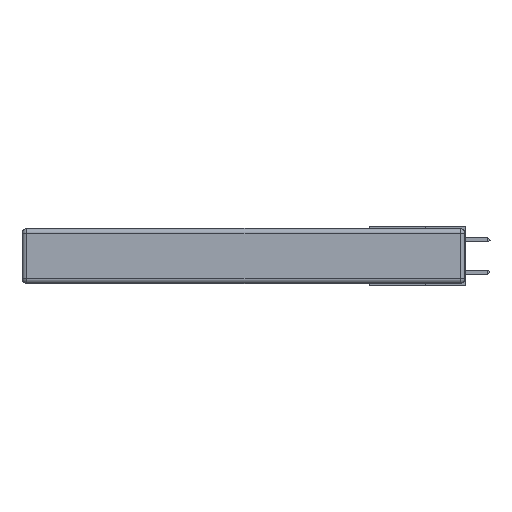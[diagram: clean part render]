
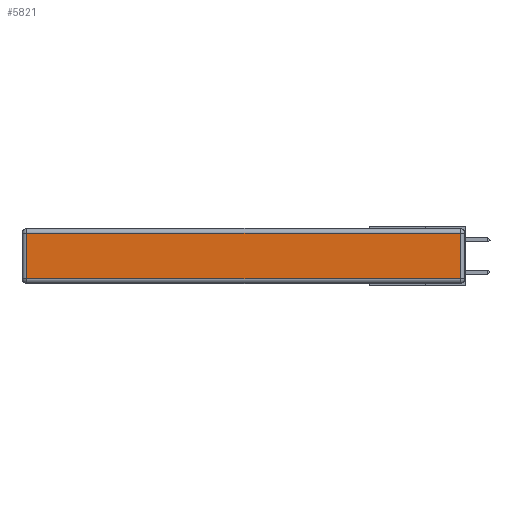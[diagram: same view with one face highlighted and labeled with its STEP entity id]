
A CAD part, left-side view. The second image highlights one B-rep face of the part: STEP entity #5821.
In plain terms, the highlighted planar face has unit normal (-1, 0, 0).
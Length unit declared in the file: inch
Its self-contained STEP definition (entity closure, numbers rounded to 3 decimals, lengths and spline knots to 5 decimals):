
#253 = DIRECTION ( 'NONE',  ( 0., 0., 1. ) ) ;
#642 = ORIENTED_EDGE ( 'NONE', *, *, #15399, .T. ) ;
#1373 = CARTESIAN_POINT ( 'NONE',  ( 0., 0., -0.313 ) ) ;
#1536 = CARTESIAN_POINT ( 'NONE',  ( 0., 0.03, -0.343 ) ) ;
#2411 = LINE ( 'NONE', #11753, #5885 ) ;
#2417 = ORIENTED_EDGE ( 'NONE', *, *, #6206, .T. ) ;
#2902 = DIRECTION ( 'NONE',  ( 0., 0., 1. ) ) ;
#4657 = AXIS2_PLACEMENT_3D ( 'NONE', #5674, #5861, #253 ) ;
#5674 = CARTESIAN_POINT ( 'NONE',  ( 0., 0., -0.343 ) ) ;
#5821 = ADVANCED_FACE ( 'NONE', ( #10409 ), #12538, .T. ) ;
#5861 = DIRECTION ( 'NONE',  ( -1., 0., 0. ) ) ;
#5885 = VECTOR ( 'NONE', #14591, 39.37008 ) ;
#6206 = EDGE_CURVE ( 'NONE', #10304, #14383, #2411, .T. ) ;
#6364 = LINE ( 'NONE', #1536, #15002 ) ;
#7269 = CARTESIAN_POINT ( 'NONE',  ( 0., 2.75, -0.03 ) ) ;
#7339 = ORIENTED_EDGE ( 'NONE', *, *, #17480, .T. ) ;
#7557 = VERTEX_POINT ( 'NONE', #16564 ) ;
#10304 = VERTEX_POINT ( 'NONE', #13798 ) ;
#10409 = FACE_OUTER_BOUND ( 'NONE', #11026, .T. ) ;
#11026 = EDGE_LOOP ( 'NONE', ( #642, #13218, #7339, #2417 ) ) ;
#11340 = EDGE_CURVE ( 'NONE', #7557, #13754, #6364, .T. ) ;
#11575 = CARTESIAN_POINT ( 'NONE',  ( 0., 2.72, -0.313 ) ) ;
#11753 = CARTESIAN_POINT ( 'NONE',  ( 0., 2.72, -0.343 ) ) ;
#12538 = PLANE ( 'NONE',  #4657 ) ;
#13218 = ORIENTED_EDGE ( 'NONE', *, *, #11340, .T. ) ;
#13429 = CARTESIAN_POINT ( 'NONE',  ( 0., 0.03, -0.03 ) ) ;
#13461 = VECTOR ( 'NONE', #14397, 39.37008 ) ;
#13754 = VERTEX_POINT ( 'NONE', #13429 ) ;
#13798 = CARTESIAN_POINT ( 'NONE',  ( 0., 2.72, -0.03 ) ) ;
#14383 = VERTEX_POINT ( 'NONE', #11575 ) ;
#14397 = DIRECTION ( 'NONE',  ( 0., 1., 0. ) ) ;
#14558 = LINE ( 'NONE', #7269, #13461 ) ;
#14591 = DIRECTION ( 'NONE',  ( 0., 0., -1. ) ) ;
#15002 = VECTOR ( 'NONE', #2902, 39.37008 ) ;
#15399 = EDGE_CURVE ( 'NONE', #14383, #7557, #16839, .T. ) ;
#16388 = VECTOR ( 'NONE', #16583, 39.37008 ) ;
#16564 = CARTESIAN_POINT ( 'NONE',  ( 0., 0.03, -0.313 ) ) ;
#16583 = DIRECTION ( 'NONE',  ( 0., -1., 0. ) ) ;
#16839 = LINE ( 'NONE', #1373, #16388 ) ;
#17480 = EDGE_CURVE ( 'NONE', #13754, #10304, #14558, .T. ) ;
